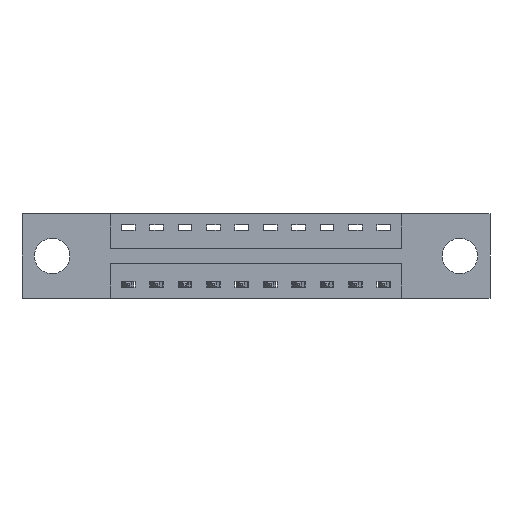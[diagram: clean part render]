
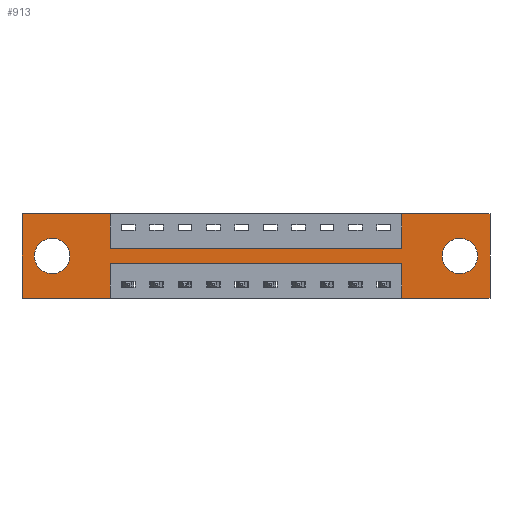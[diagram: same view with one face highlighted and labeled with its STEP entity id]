
A CAD part, front view. The second image highlights one B-rep face of the part: STEP entity #913.
In plain terms, the highlighted planar face has unit normal (0, -1, 0).
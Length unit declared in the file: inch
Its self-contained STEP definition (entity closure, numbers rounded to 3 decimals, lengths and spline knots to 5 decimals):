
#159 = VECTOR ( 'NONE', #1774, 39.37008 ) ;
#201 = DIRECTION ( 'NONE',  ( 0., 0., 1. ) ) ;
#230 = EDGE_CURVE ( 'NONE', #5587, #6515, #7935, .T. ) ;
#387 = ORIENTED_EDGE ( 'NONE', *, *, #8654, .F. ) ;
#452 = VERTEX_POINT ( 'NONE', #2228 ) ;
#515 = AXIS2_PLACEMENT_3D ( 'NONE', #8875, #4031, #9670 ) ;
#535 = VERTEX_POINT ( 'NONE', #5624 ) ;
#694 = VERTEX_POINT ( 'NONE', #8446 ) ;
#762 = VECTOR ( 'NONE', #7137, 39.37008 ) ;
#821 = EDGE_LOOP ( 'NONE', ( #3655, #6655 ) ) ;
#870 = CARTESIAN_POINT ( 'NONE',  ( 0.1325, 0., -0.263 ) ) ;
#883 = EDGE_LOOP ( 'NONE', ( #10094, #7968 ) ) ;
#903 = VERTEX_POINT ( 'NONE', #6975 ) ;
#913 = ADVANCED_FACE ( 'NONE', ( #10414, #8045, #3729 ), #7961, .T. ) ;
#970 = ORIENTED_EDGE ( 'NONE', *, *, #1903, .F. ) ;
#1058 = CARTESIAN_POINT ( 'NONE',  ( 0., 0., -0.37 ) ) ;
#1073 = DIRECTION ( 'NONE',  ( 1., 0., 0. ) ) ;
#1199 = EDGE_CURVE ( 'NONE', #7869, #535, #7162, .T. ) ;
#1247 = CARTESIAN_POINT ( 'NONE',  ( 0., 0., 0. ) ) ;
#1268 = DIRECTION ( 'NONE',  ( 0., 0., 1. ) ) ;
#1286 = DIRECTION ( 'NONE',  ( 0., 1., 0. ) ) ;
#1375 = CIRCLE ( 'NONE', #4821, 0.078 ) ;
#1388 = CARTESIAN_POINT ( 'NONE',  ( 2.06, 0., 0. ) ) ;
#1479 = CARTESIAN_POINT ( 'NONE',  ( 0.3875, 0., -0.37 ) ) ;
#1497 = EDGE_LOOP ( 'NONE', ( #387, #4714, #5550, #5021, #970, #1877, #9672, #4610, #4010, #9390, #6060, #1667 ) ) ;
#1557 = CARTESIAN_POINT ( 'NONE',  ( 0.3875, 0., 0. ) ) ;
#1636 = EDGE_CURVE ( 'NONE', #6515, #7216, #7662, .T. ) ;
#1667 = ORIENTED_EDGE ( 'NONE', *, *, #8523, .F. ) ;
#1679 = VECTOR ( 'NONE', #6779, 39.37008 ) ;
#1735 = CARTESIAN_POINT ( 'NONE',  ( 1.6725, 0., -0.15 ) ) ;
#1774 = DIRECTION ( 'NONE',  ( 0., 0., 1. ) ) ;
#1877 = ORIENTED_EDGE ( 'NONE', *, *, #2889, .F. ) ;
#1903 = EDGE_CURVE ( 'NONE', #4137, #7869, #7277, .T. ) ;
#1927 = LINE ( 'NONE', #5929, #1679 ) ;
#2024 = LINE ( 'NONE', #1557, #4473 ) ;
#2228 = CARTESIAN_POINT ( 'NONE',  ( 0.3875, 0., -0.22 ) ) ;
#2505 = CARTESIAN_POINT ( 'NONE',  ( 0.3875, 0., 0. ) ) ;
#2638 = EDGE_CURVE ( 'NONE', #3384, #5587, #2024, .T. ) ;
#2724 = VERTEX_POINT ( 'NONE', #6524 ) ;
#2735 = VERTEX_POINT ( 'NONE', #870 ) ;
#2857 = DIRECTION ( 'NONE',  ( 1., 0., 0. ) ) ;
#2874 = EDGE_CURVE ( 'NONE', #2724, #2735, #8126, .T. ) ;
#2889 = EDGE_CURVE ( 'NONE', #7216, #4137, #10251, .T. ) ;
#2939 = VECTOR ( 'NONE', #7187, 39.37008 ) ;
#2990 = EDGE_CURVE ( 'NONE', #2735, #2724, #1375, .T. ) ;
#3000 = VERTEX_POINT ( 'NONE', #10127 ) ;
#3029 = VECTOR ( 'NONE', #201, 39.37008 ) ;
#3191 = LINE ( 'NONE', #1479, #2939 ) ;
#3384 = VERTEX_POINT ( 'NONE', #2505 ) ;
#3564 = CARTESIAN_POINT ( 'NONE',  ( 2.06, 0., 0. ) ) ;
#3572 = CARTESIAN_POINT ( 'NONE',  ( 1.6725, 0., 0. ) ) ;
#3614 = VECTOR ( 'NONE', #4963, 39.37008 ) ;
#3641 = CARTESIAN_POINT ( 'NONE',  ( 2.06, 0., -0.37 ) ) ;
#3655 = ORIENTED_EDGE ( 'NONE', *, *, #2874, .T. ) ;
#3658 = CARTESIAN_POINT ( 'NONE',  ( 0.1325, 0., -0.185 ) ) ;
#3729 = FACE_OUTER_BOUND ( 'NONE', #1497, .T. ) ;
#3774 = DIRECTION ( 'NONE',  ( -1., 0., 0. ) ) ;
#3787 = VECTOR ( 'NONE', #2857, 39.37008 ) ;
#3813 = VECTOR ( 'NONE', #1073, 39.37008 ) ;
#3948 = DIRECTION ( 'NONE',  ( -1., 0., 0. ) ) ;
#4010 = ORIENTED_EDGE ( 'NONE', *, *, #2638, .F. ) ;
#4031 = DIRECTION ( 'NONE',  ( 0., 1., 0. ) ) ;
#4035 = LINE ( 'NONE', #6669, #159 ) ;
#4036 = CARTESIAN_POINT ( 'NONE',  ( 0.3875, 0., -0.37 ) ) ;
#4137 = VERTEX_POINT ( 'NONE', #3564 ) ;
#4352 = CARTESIAN_POINT ( 'NONE',  ( 0.1325, 0., -0.185 ) ) ;
#4456 = CARTESIAN_POINT ( 'NONE',  ( 1.9275, 0., -0.263 ) ) ;
#4473 = VECTOR ( 'NONE', #7261, 39.37008 ) ;
#4499 = DIRECTION ( 'NONE',  ( 0., 0., 1. ) ) ;
#4500 = LINE ( 'NONE', #5418, #8278 ) ;
#4610 = ORIENTED_EDGE ( 'NONE', *, *, #230, .F. ) ;
#4714 = ORIENTED_EDGE ( 'NONE', *, *, #8306, .F. ) ;
#4723 = EDGE_CURVE ( 'NONE', #535, #3000, #5223, .T. ) ;
#4821 = AXIS2_PLACEMENT_3D ( 'NONE', #3658, #9314, #4499 ) ;
#4885 = VERTEX_POINT ( 'NONE', #4456 ) ;
#4963 = DIRECTION ( 'NONE',  ( 1., 0., 0. ) ) ;
#5016 = VECTOR ( 'NONE', #3948, 39.37008 ) ;
#5021 = ORIENTED_EDGE ( 'NONE', *, *, #1199, .F. ) ;
#5135 = CARTESIAN_POINT ( 'NONE',  ( 1.6725, 0., -0.37 ) ) ;
#5171 = DIRECTION ( 'NONE',  ( 0., 0., 1. ) ) ;
#5223 = LINE ( 'NONE', #5135, #3029 ) ;
#5418 = CARTESIAN_POINT ( 'NONE',  ( 0., 0., -0.37 ) ) ;
#5529 = EDGE_CURVE ( 'NONE', #9137, #3384, #5691, .T. ) ;
#5550 = ORIENTED_EDGE ( 'NONE', *, *, #4723, .F. ) ;
#5587 = VERTEX_POINT ( 'NONE', #7767 ) ;
#5624 = CARTESIAN_POINT ( 'NONE',  ( 1.6725, 0., -0.37 ) ) ;
#5691 = LINE ( 'NONE', #7733, #3787 ) ;
#5783 = AXIS2_PLACEMENT_3D ( 'NONE', #6181, #1286, #7014 ) ;
#5929 = CARTESIAN_POINT ( 'NONE',  ( 0.3875, 0., -0.22 ) ) ;
#6060 = ORIENTED_EDGE ( 'NONE', *, *, #10177, .F. ) ;
#6181 = CARTESIAN_POINT ( 'NONE',  ( 1.9275, 0., -0.185 ) ) ;
#6350 = EDGE_CURVE ( 'NONE', #4885, #694, #6451, .T. ) ;
#6451 = CIRCLE ( 'NONE', #515, 0.078 ) ;
#6515 = VERTEX_POINT ( 'NONE', #1735 ) ;
#6524 = CARTESIAN_POINT ( 'NONE',  ( 0.1325, 0., -0.107 ) ) ;
#6655 = ORIENTED_EDGE ( 'NONE', *, *, #2990, .T. ) ;
#6669 = CARTESIAN_POINT ( 'NONE',  ( 0., 0., 0. ) ) ;
#6764 = EDGE_CURVE ( 'NONE', #694, #4885, #9073, .T. ) ;
#6779 = DIRECTION ( 'NONE',  ( -1., 0., 0. ) ) ;
#6975 = CARTESIAN_POINT ( 'NONE',  ( 0., 0., -0.37 ) ) ;
#7014 = DIRECTION ( 'NONE',  ( 0., 0., -1. ) ) ;
#7137 = DIRECTION ( 'NONE',  ( 0., 0., -1. ) ) ;
#7162 = LINE ( 'NONE', #1058, #5016 ) ;
#7187 = DIRECTION ( 'NONE',  ( 0., 0., -1. ) ) ;
#7216 = VERTEX_POINT ( 'NONE', #3572 ) ;
#7257 = CARTESIAN_POINT ( 'NONE',  ( 1.6725, 0., 0. ) ) ;
#7261 = DIRECTION ( 'NONE',  ( 0., 0., -1. ) ) ;
#7277 = LINE ( 'NONE', #1388, #762 ) ;
#7312 = AXIS2_PLACEMENT_3D ( 'NONE', #9703, #8823, #9802 ) ;
#7662 = LINE ( 'NONE', #7257, #10034 ) ;
#7733 = CARTESIAN_POINT ( 'NONE',  ( 0., 0., 0. ) ) ;
#7767 = CARTESIAN_POINT ( 'NONE',  ( 0.3875, 0., -0.15 ) ) ;
#7869 = VERTEX_POINT ( 'NONE', #3641 ) ;
#7935 = LINE ( 'NONE', #10008, #3614 ) ;
#7961 = PLANE ( 'NONE',  #7312 ) ;
#7968 = ORIENTED_EDGE ( 'NONE', *, *, #6350, .T. ) ;
#8045 = FACE_BOUND ( 'NONE', #821, .T. ) ;
#8126 = CIRCLE ( 'NONE', #9871, 0.078 ) ;
#8215 = VERTEX_POINT ( 'NONE', #4036 ) ;
#8278 = VECTOR ( 'NONE', #3774, 39.37008 ) ;
#8306 = EDGE_CURVE ( 'NONE', #3000, #452, #1927, .T. ) ;
#8374 = CARTESIAN_POINT ( 'NONE',  ( 0., 0., 0. ) ) ;
#8446 = CARTESIAN_POINT ( 'NONE',  ( 1.9275, 0., -0.107 ) ) ;
#8523 = EDGE_CURVE ( 'NONE', #8215, #903, #4500, .T. ) ;
#8654 = EDGE_CURVE ( 'NONE', #452, #8215, #3191, .T. ) ;
#8823 = DIRECTION ( 'NONE',  ( 0., -1., 0. ) ) ;
#8875 = CARTESIAN_POINT ( 'NONE',  ( 1.9275, 0., -0.185 ) ) ;
#9073 = CIRCLE ( 'NONE', #5783, 0.078 ) ;
#9137 = VERTEX_POINT ( 'NONE', #1247 ) ;
#9314 = DIRECTION ( 'NONE',  ( 0., 1., 0. ) ) ;
#9390 = ORIENTED_EDGE ( 'NONE', *, *, #5529, .F. ) ;
#9670 = DIRECTION ( 'NONE',  ( 0., 0., -1. ) ) ;
#9672 = ORIENTED_EDGE ( 'NONE', *, *, #1636, .F. ) ;
#9703 = CARTESIAN_POINT ( 'NONE',  ( 0., 0., -0.37 ) ) ;
#9802 = DIRECTION ( 'NONE',  ( 0., 0., -1. ) ) ;
#9871 = AXIS2_PLACEMENT_3D ( 'NONE', #4352, #9980, #5171 ) ;
#9980 = DIRECTION ( 'NONE',  ( 0., 1., 0. ) ) ;
#10008 = CARTESIAN_POINT ( 'NONE',  ( 0.3875, 0., -0.15 ) ) ;
#10034 = VECTOR ( 'NONE', #1268, 39.37008 ) ;
#10094 = ORIENTED_EDGE ( 'NONE', *, *, #6764, .T. ) ;
#10127 = CARTESIAN_POINT ( 'NONE',  ( 1.6725, 0., -0.22 ) ) ;
#10177 = EDGE_CURVE ( 'NONE', #903, #9137, #4035, .T. ) ;
#10251 = LINE ( 'NONE', #8374, #3813 ) ;
#10414 = FACE_BOUND ( 'NONE', #883, .T. ) ;
